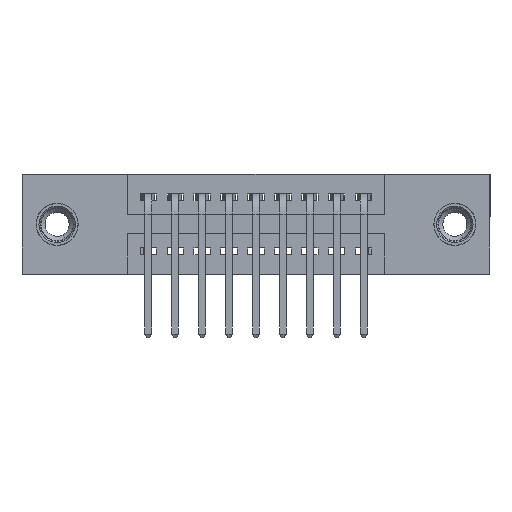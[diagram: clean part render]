
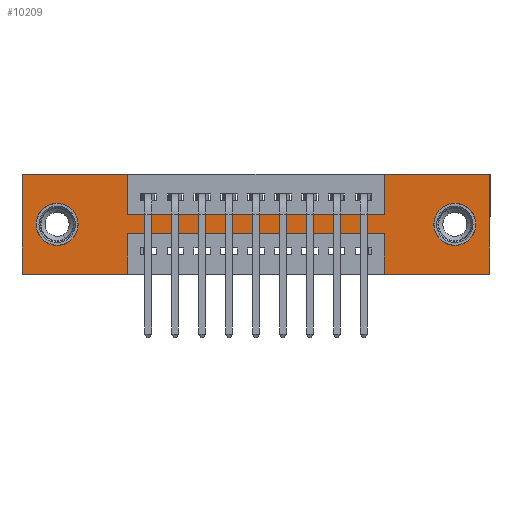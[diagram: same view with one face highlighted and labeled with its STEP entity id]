
A CAD part, front view. The second image highlights one B-rep face of the part: STEP entity #10209.
In plain terms, the highlighted planar face has unit normal (0, -1, 0).
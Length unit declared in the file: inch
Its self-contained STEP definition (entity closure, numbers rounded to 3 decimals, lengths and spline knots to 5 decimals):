
#49 = VERTEX_POINT ( 'NONE', #11936 ) ;
#370 = VERTEX_POINT ( 'NONE', #14210 ) ;
#398 = ORIENTED_EDGE ( 'NONE', *, *, #3318, .F. ) ;
#415 = AXIS2_PLACEMENT_3D ( 'NONE', #4313, #13121, #5670 ) ;
#599 = ORIENTED_EDGE ( 'NONE', *, *, #6691, .F. ) ;
#684 = CIRCLE ( 'NONE', #11145, 0.078 ) ;
#981 = AXIS2_PLACEMENT_3D ( 'NONE', #4569, #13347, #5922 ) ;
#992 = DIRECTION ( 'NONE',  ( 0., 0., -1. ) ) ;
#1018 = LINE ( 'NONE', #2114, #14041 ) ;
#1321 = CARTESIAN_POINT ( 'NONE',  ( 1.3425, 0., 0. ) ) ;
#1463 = CARTESIAN_POINT ( 'NONE',  ( 0., 0., 0. ) ) ;
#1701 = CARTESIAN_POINT ( 'NONE',  ( 0., 0., 0. ) ) ;
#1830 = VECTOR ( 'NONE', #8321, 39.37008 ) ;
#2076 = CARTESIAN_POINT ( 'NONE',  ( 0., 0., -0.37 ) ) ;
#2114 = CARTESIAN_POINT ( 'NONE',  ( 0., 0., -0.37 ) ) ;
#2228 = EDGE_CURVE ( 'NONE', #49, #4353, #4636, .T. ) ;
#2284 = CARTESIAN_POINT ( 'NONE',  ( 0.3925, 0., 0. ) ) ;
#2400 = ORIENTED_EDGE ( 'NONE', *, *, #14637, .T. ) ;
#2675 = LINE ( 'NONE', #12047, #8887 ) ;
#2684 = DIRECTION ( 'NONE',  ( 0., 0., -1. ) ) ;
#3318 = EDGE_CURVE ( 'NONE', #4210, #8548, #14470, .T. ) ;
#3840 = EDGE_CURVE ( 'NONE', #14534, #9509, #8512, .T. ) ;
#3923 = CARTESIAN_POINT ( 'NONE',  ( 1.3425, 0., -0.37 ) ) ;
#4007 = CARTESIAN_POINT ( 'NONE',  ( 0., 0., 0. ) ) ;
#4210 = VERTEX_POINT ( 'NONE', #6915 ) ;
#4264 = VERTEX_POINT ( 'NONE', #14393 ) ;
#4313 = CARTESIAN_POINT ( 'NONE',  ( 0.13, 0., -0.185 ) ) ;
#4353 = VERTEX_POINT ( 'NONE', #7358 ) ;
#4545 = VECTOR ( 'NONE', #8808, 39.37008 ) ;
#4569 = CARTESIAN_POINT ( 'NONE',  ( 1.605, 0., -0.185 ) ) ;
#4636 = LINE ( 'NONE', #2284, #14154 ) ;
#5007 = VECTOR ( 'NONE', #12265, 39.37008 ) ;
#5024 = VECTOR ( 'NONE', #10654, 39.37008 ) ;
#5403 = EDGE_LOOP ( 'NONE', ( #15229, #2400 ) ) ;
#5518 = DIRECTION ( 'NONE',  ( 0., 1., 0. ) ) ;
#5670 = DIRECTION ( 'NONE',  ( 0., 0., 1. ) ) ;
#5691 = CARTESIAN_POINT ( 'NONE',  ( 1.735, 0., 0. ) ) ;
#5732 = DIRECTION ( 'NONE',  ( 1., 0., 0. ) ) ;
#5854 = VERTEX_POINT ( 'NONE', #7033 ) ;
#5922 = DIRECTION ( 'NONE',  ( 0., 0., -1. ) ) ;
#6073 = EDGE_CURVE ( 'NONE', #13701, #4210, #1018, .T. ) ;
#6227 = AXIS2_PLACEMENT_3D ( 'NONE', #10382, #10435, #2684 ) ;
#6240 = VERTEX_POINT ( 'NONE', #11333 ) ;
#6475 = FACE_OUTER_BOUND ( 'NONE', #12513, .T. ) ;
#6691 = EDGE_CURVE ( 'NONE', #7605, #13144, #8853, .T. ) ;
#6755 = ORIENTED_EDGE ( 'NONE', *, *, #3840, .F. ) ;
#6784 = CIRCLE ( 'NONE', #7481, 0.078 ) ;
#6915 = CARTESIAN_POINT ( 'NONE',  ( 0., 0., -0.37 ) ) ;
#7033 = CARTESIAN_POINT ( 'NONE',  ( 1.605, 0., -0.263 ) ) ;
#7042 = EDGE_LOOP ( 'NONE', ( #8609, #11788 ) ) ;
#7204 = DIRECTION ( 'NONE',  ( 0., 0., -1. ) ) ;
#7358 = CARTESIAN_POINT ( 'NONE',  ( 0.3925, 0., -0.15 ) ) ;
#7381 = ORIENTED_EDGE ( 'NONE', *, *, #6073, .F. ) ;
#7462 = CIRCLE ( 'NONE', #415, 0.078 ) ;
#7481 = AXIS2_PLACEMENT_3D ( 'NONE', #14959, #7803, #16032 ) ;
#7485 = CARTESIAN_POINT ( 'NONE',  ( 1.3425, 0., -0.37 ) ) ;
#7605 = VERTEX_POINT ( 'NONE', #1321 ) ;
#7803 = DIRECTION ( 'NONE',  ( 0., 1., 0. ) ) ;
#7804 = VECTOR ( 'NONE', #10496, 39.37008 ) ;
#7874 = CARTESIAN_POINT ( 'NONE',  ( 0.3925, 0., -0.22 ) ) ;
#8014 = VECTOR ( 'NONE', #14820, 39.37008 ) ;
#8321 = DIRECTION ( 'NONE',  ( 0., 0., -1. ) ) ;
#8450 = VECTOR ( 'NONE', #8665, 39.37008 ) ;
#8512 = LINE ( 'NONE', #2076, #5007 ) ;
#8548 = VERTEX_POINT ( 'NONE', #4007 ) ;
#8609 = ORIENTED_EDGE ( 'NONE', *, *, #10998, .T. ) ;
#8665 = DIRECTION ( 'NONE',  ( 1., 0., 0. ) ) ;
#8808 = DIRECTION ( 'NONE',  ( 0., 0., 1. ) ) ;
#8853 = LINE ( 'NONE', #12231, #8450 ) ;
#8887 = VECTOR ( 'NONE', #7204, 39.37008 ) ;
#8946 = CARTESIAN_POINT ( 'NONE',  ( 1.3425, 0., 0. ) ) ;
#9239 = PLANE ( 'NONE',  #6227 ) ;
#9509 = VERTEX_POINT ( 'NONE', #3923 ) ;
#9561 = ORIENTED_EDGE ( 'NONE', *, *, #2228, .F. ) ;
#9597 = CARTESIAN_POINT ( 'NONE',  ( 0.3925, 0., -0.15 ) ) ;
#9640 = VECTOR ( 'NONE', #12654, 39.37008 ) ;
#9737 = VECTOR ( 'NONE', #5732, 39.37008 ) ;
#9738 = ORIENTED_EDGE ( 'NONE', *, *, #12610, .F. ) ;
#10209 = ADVANCED_FACE ( 'NONE', ( #13056, #15998, #6475 ), #9239, .T. ) ;
#10382 = CARTESIAN_POINT ( 'NONE',  ( 0., 0., -0.37 ) ) ;
#10435 = DIRECTION ( 'NONE',  ( 0., -1., 0. ) ) ;
#10496 = DIRECTION ( 'NONE',  ( 1., 0., 0. ) ) ;
#10635 = VERTEX_POINT ( 'NONE', #12147 ) ;
#10643 = VERTEX_POINT ( 'NONE', #15639 ) ;
#10654 = DIRECTION ( 'NONE',  ( 0., 0., 1. ) ) ;
#10998 = EDGE_CURVE ( 'NONE', #4264, #5854, #684, .T. ) ;
#11050 = LINE ( 'NONE', #1463, #7804 ) ;
#11072 = DIRECTION ( 'NONE',  ( -1., 0., 0. ) ) ;
#11145 = AXIS2_PLACEMENT_3D ( 'NONE', #12978, #5518, #14143 ) ;
#11221 = ORIENTED_EDGE ( 'NONE', *, *, #14553, .F. ) ;
#11248 = LINE ( 'NONE', #8946, #8014 ) ;
#11274 = CARTESIAN_POINT ( 'NONE',  ( 1.735, 0., -0.37 ) ) ;
#11333 = CARTESIAN_POINT ( 'NONE',  ( 0.13, 0., -0.263 ) ) ;
#11662 = LINE ( 'NONE', #7485, #4545 ) ;
#11788 = ORIENTED_EDGE ( 'NONE', *, *, #15102, .T. ) ;
#11794 = EDGE_CURVE ( 'NONE', #370, #6240, #7462, .T. ) ;
#11880 = EDGE_CURVE ( 'NONE', #13768, #13701, #2675, .T. ) ;
#11936 = CARTESIAN_POINT ( 'NONE',  ( 0.3925, 0., 0. ) ) ;
#11987 = ORIENTED_EDGE ( 'NONE', *, *, #15642, .F. ) ;
#11998 = LINE ( 'NONE', #5691, #1830 ) ;
#12047 = CARTESIAN_POINT ( 'NONE',  ( 0.3925, 0., -0.37 ) ) ;
#12147 = CARTESIAN_POINT ( 'NONE',  ( 1.3425, 0., -0.15 ) ) ;
#12231 = CARTESIAN_POINT ( 'NONE',  ( 0., 0., 0. ) ) ;
#12265 = DIRECTION ( 'NONE',  ( -1., 0., 0. ) ) ;
#12513 = EDGE_LOOP ( 'NONE', ( #15572, #9738, #15899, #6755, #13676, #599, #11221, #11987, #9561, #13501, #398, #7381 ) ) ;
#12610 = EDGE_CURVE ( 'NONE', #10643, #13768, #12841, .T. ) ;
#12654 = DIRECTION ( 'NONE',  ( -1., 0., 0. ) ) ;
#12841 = LINE ( 'NONE', #15986, #9640 ) ;
#12978 = CARTESIAN_POINT ( 'NONE',  ( 1.605, 0., -0.185 ) ) ;
#13056 = FACE_BOUND ( 'NONE', #7042, .T. ) ;
#13121 = DIRECTION ( 'NONE',  ( 0., 1., 0. ) ) ;
#13144 = VERTEX_POINT ( 'NONE', #14848 ) ;
#13332 = CIRCLE ( 'NONE', #981, 0.078 ) ;
#13347 = DIRECTION ( 'NONE',  ( 0., 1., 0. ) ) ;
#13501 = ORIENTED_EDGE ( 'NONE', *, *, #14805, .F. ) ;
#13505 = EDGE_CURVE ( 'NONE', #9509, #10643, #11662, .T. ) ;
#13676 = ORIENTED_EDGE ( 'NONE', *, *, #14960, .F. ) ;
#13701 = VERTEX_POINT ( 'NONE', #13812 ) ;
#13768 = VERTEX_POINT ( 'NONE', #7874 ) ;
#13812 = CARTESIAN_POINT ( 'NONE',  ( 0.3925, 0., -0.37 ) ) ;
#14041 = VECTOR ( 'NONE', #11072, 39.37008 ) ;
#14143 = DIRECTION ( 'NONE',  ( 0., 0., -1. ) ) ;
#14154 = VECTOR ( 'NONE', #992, 39.37008 ) ;
#14210 = CARTESIAN_POINT ( 'NONE',  ( 0.13, 0., -0.107 ) ) ;
#14393 = CARTESIAN_POINT ( 'NONE',  ( 1.605, 0., -0.107 ) ) ;
#14470 = LINE ( 'NONE', #1701, #5024 ) ;
#14534 = VERTEX_POINT ( 'NONE', #11274 ) ;
#14553 = EDGE_CURVE ( 'NONE', #10635, #7605, #11248, .T. ) ;
#14637 = EDGE_CURVE ( 'NONE', #6240, #370, #6784, .T. ) ;
#14805 = EDGE_CURVE ( 'NONE', #8548, #49, #11050, .T. ) ;
#14820 = DIRECTION ( 'NONE',  ( 0., 0., 1. ) ) ;
#14848 = CARTESIAN_POINT ( 'NONE',  ( 1.735, 0., 0. ) ) ;
#14959 = CARTESIAN_POINT ( 'NONE',  ( 0.13, 0., -0.185 ) ) ;
#14960 = EDGE_CURVE ( 'NONE', #13144, #14534, #11998, .T. ) ;
#15102 = EDGE_CURVE ( 'NONE', #5854, #4264, #13332, .T. ) ;
#15229 = ORIENTED_EDGE ( 'NONE', *, *, #11794, .T. ) ;
#15572 = ORIENTED_EDGE ( 'NONE', *, *, #11880, .F. ) ;
#15639 = CARTESIAN_POINT ( 'NONE',  ( 1.3425, 0., -0.22 ) ) ;
#15642 = EDGE_CURVE ( 'NONE', #4353, #10635, #15898, .T. ) ;
#15898 = LINE ( 'NONE', #9597, #9737 ) ;
#15899 = ORIENTED_EDGE ( 'NONE', *, *, #13505, .F. ) ;
#15986 = CARTESIAN_POINT ( 'NONE',  ( 0.3925, 0., -0.22 ) ) ;
#15998 = FACE_BOUND ( 'NONE', #5403, .T. ) ;
#16032 = DIRECTION ( 'NONE',  ( 0., 0., 1. ) ) ;
